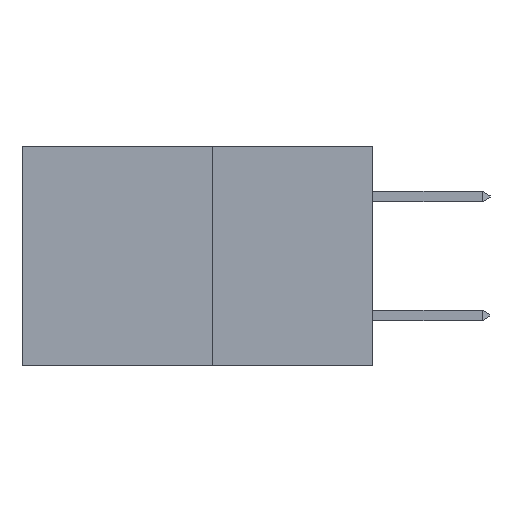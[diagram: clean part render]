
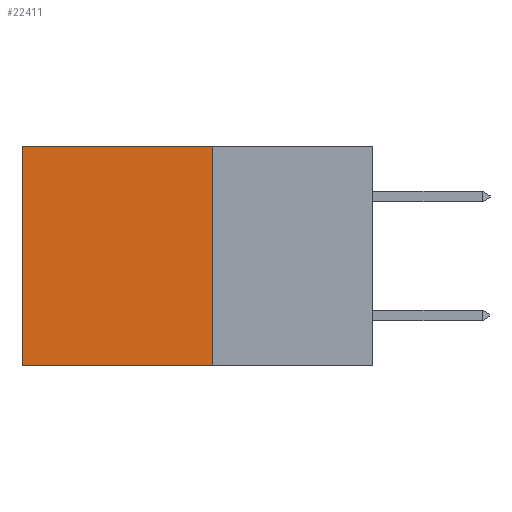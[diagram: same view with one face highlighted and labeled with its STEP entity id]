
A CAD part, left-side view. The second image highlights one B-rep face of the part: STEP entity #22411.
In plain terms, the highlighted planar face has unit normal (-1, 0, 0).
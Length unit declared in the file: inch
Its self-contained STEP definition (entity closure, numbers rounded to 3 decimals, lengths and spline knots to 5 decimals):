
#180 = VECTOR ( 'NONE', #3304, 39.37008 ) ;
#299 = VECTOR ( 'NONE', #908, 39.37008 ) ;
#858 = CARTESIAN_POINT ( 'NONE',  ( 0.277, 0.27, 0. ) ) ;
#908 = DIRECTION ( 'NONE',  ( 0., 1., 0. ) ) ;
#1140 = EDGE_CURVE ( 'NONE', #7786, #8217, #6877, .T. ) ;
#1670 = DIRECTION ( 'NONE',  ( 0., 0., -1. ) ) ;
#3304 = DIRECTION ( 'NONE',  ( 0., 1., 0. ) ) ;
#3835 = ORIENTED_EDGE ( 'NONE', *, *, #26412, .T. ) ;
#4432 = VERTEX_POINT ( 'NONE', #19101 ) ;
#5250 = ORIENTED_EDGE ( 'NONE', *, *, #28051, .T. ) ;
#6877 = LINE ( 'NONE', #18193, #299 ) ;
#7786 = VERTEX_POINT ( 'NONE', #11300 ) ;
#8217 = VERTEX_POINT ( 'NONE', #28123 ) ;
#8521 = ORIENTED_EDGE ( 'NONE', *, *, #1140, .F. ) ;
#8986 = AXIS2_PLACEMENT_3D ( 'NONE', #13904, #16382, #1670 ) ;
#9734 = VECTOR ( 'NONE', #18531, 39.37008 ) ;
#11300 = CARTESIAN_POINT ( 'NONE',  ( 0.277, 0.27, -0.37 ) ) ;
#13499 = CARTESIAN_POINT ( 'NONE',  ( 0.277, 0.59, -0.37 ) ) ;
#13904 = CARTESIAN_POINT ( 'NONE',  ( 0.277, 0.27, -0.37 ) ) ;
#14032 = LINE ( 'NONE', #858, #180 ) ;
#15688 = VERTEX_POINT ( 'NONE', #21625 ) ;
#16044 = ORIENTED_EDGE ( 'NONE', *, *, #25631, .F. ) ;
#16382 = DIRECTION ( 'NONE',  ( 1., 0., 0. ) ) ;
#16790 = VECTOR ( 'NONE', #27094, 39.37008 ) ;
#18193 = CARTESIAN_POINT ( 'NONE',  ( 0.277, 0.27, -0.37 ) ) ;
#18531 = DIRECTION ( 'NONE',  ( 0., 0., -1. ) ) ;
#19101 = CARTESIAN_POINT ( 'NONE',  ( 0.277, 0.59, 0. ) ) ;
#21625 = CARTESIAN_POINT ( 'NONE',  ( 0.277, 0.27, 0. ) ) ;
#22233 = CARTESIAN_POINT ( 'NONE',  ( 0.277, 0.27, -0.37 ) ) ;
#22411 = ADVANCED_FACE ( 'NONE', ( #28321 ), #28459, .F. ) ;
#25631 = EDGE_CURVE ( 'NONE', #15688, #7786, #28923, .T. ) ;
#26412 = EDGE_CURVE ( 'NONE', #15688, #4432, #14032, .T. ) ;
#27094 = DIRECTION ( 'NONE',  ( 0., 0., -1. ) ) ;
#28051 = EDGE_CURVE ( 'NONE', #4432, #8217, #29155, .T. ) ;
#28123 = CARTESIAN_POINT ( 'NONE',  ( 0.277, 0.59, -0.37 ) ) ;
#28321 = FACE_OUTER_BOUND ( 'NONE', #30967, .T. ) ;
#28459 = PLANE ( 'NONE',  #8986 ) ;
#28923 = LINE ( 'NONE', #22233, #16790 ) ;
#29155 = LINE ( 'NONE', #13499, #9734 ) ;
#30967 = EDGE_LOOP ( 'NONE', ( #5250, #8521, #16044, #3835 ) ) ;
